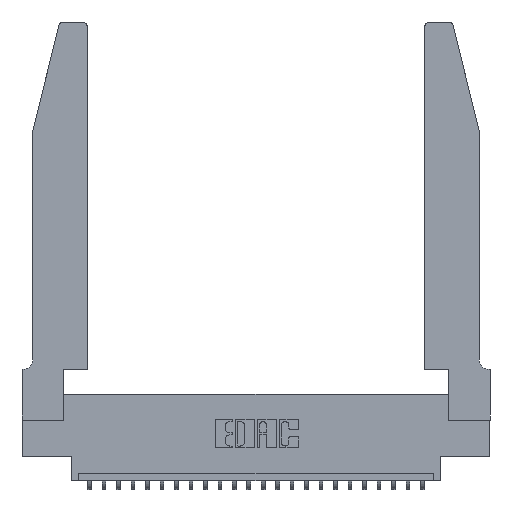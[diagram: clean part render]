
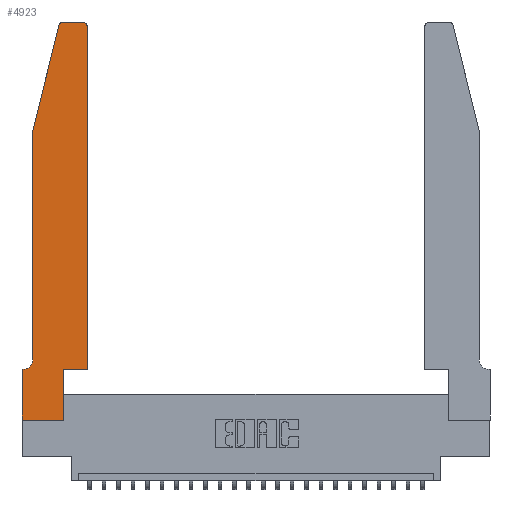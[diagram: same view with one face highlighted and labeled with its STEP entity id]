
A CAD part, top view. The second image highlights one B-rep face of the part: STEP entity #4923.
In plain terms, the highlighted planar face has unit normal (0, 0, 1).
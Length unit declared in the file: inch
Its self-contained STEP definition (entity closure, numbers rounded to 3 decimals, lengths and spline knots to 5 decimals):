
#191 = VERTEX_POINT ( 'NONE', #4531 ) ;
#282 = ORIENTED_EDGE ( 'NONE', *, *, #14211, .T. ) ;
#309 = CARTESIAN_POINT ( 'NONE',  ( 0.284, 2.72, 0.37 ) ) ;
#685 = VERTEX_POINT ( 'NONE', #8182 ) ;
#1137 = CARTESIAN_POINT ( 'NONE',  ( 0.4505, 0.35, 0.37 ) ) ;
#1182 = VERTEX_POINT ( 'NONE', #21952 ) ;
#1491 = CARTESIAN_POINT ( 'NONE',  ( 0.25487, 2.72718, 0.37 ) ) ;
#1698 = CARTESIAN_POINT ( 'NONE',  ( 0.4505, 0.35, 0.37 ) ) ;
#2178 = ORIENTED_EDGE ( 'NONE', *, *, #23063, .T. ) ;
#2293 = DIRECTION ( 'NONE',  ( 1., 0., 0. ) ) ;
#2399 = DIRECTION ( 'NONE',  ( -0.239, -0.971, 0. ) ) ;
#2492 = EDGE_CURVE ( 'NONE', #14007, #6624, #25092, .T. ) ;
#2654 = AXIS2_PLACEMENT_3D ( 'NONE', #11198, #19302, #3486 ) ;
#2881 = DIRECTION ( 'NONE',  ( -1., 0., 0. ) ) ;
#3036 = ORIENTED_EDGE ( 'NONE', *, *, #6409, .T. ) ;
#3486 = DIRECTION ( 'NONE',  ( 1., 0., 0. ) ) ;
#3730 = CIRCLE ( 'NONE', #21318, 0.03 ) ;
#4448 = DIRECTION ( 'NONE',  ( 0., 0., 1. ) ) ;
#4531 = CARTESIAN_POINT ( 'NONE',  ( 0.0755, 0.42, 0.37 ) ) ;
#4923 = ADVANCED_FACE ( 'NONE', ( #9296 ), #25029, .T. ) ;
#5009 = CARTESIAN_POINT ( 'NONE',  ( 0.0055, 0.42, 0.37 ) ) ;
#5676 = EDGE_CURVE ( 'NONE', #8826, #8177, #3730, .T. ) ;
#5836 = VERTEX_POINT ( 'NONE', #19314 ) ;
#6195 = DIRECTION ( 'NONE',  ( 0., 0., 1. ) ) ;
#6409 = EDGE_CURVE ( 'NONE', #7319, #21536, #24870, .T. ) ;
#6624 = VERTEX_POINT ( 'NONE', #1491 ) ;
#7091 = CARTESIAN_POINT ( 'NONE',  ( 0., 0.35, 0.37 ) ) ;
#7319 = VERTEX_POINT ( 'NONE', #7091 ) ;
#7355 = EDGE_LOOP ( 'NONE', ( #13079, #23089, #7685, #14093, #282, #2178, #3036, #17144, #7755, #24000, #13424, #10291 ) ) ;
#7619 = VECTOR ( 'NONE', #20845, 39.37008 ) ;
#7685 = ORIENTED_EDGE ( 'NONE', *, *, #12689, .T. ) ;
#7755 = ORIENTED_EDGE ( 'NONE', *, *, #13783, .T. ) ;
#7834 = DIRECTION ( 'NONE',  ( 0., 1., 0. ) ) ;
#8177 = VERTEX_POINT ( 'NONE', #15649 ) ;
#8182 = CARTESIAN_POINT ( 'NONE',  ( 0.4505, 0.35, 0.37 ) ) ;
#8200 = LINE ( 'NONE', #14822, #7619 ) ;
#8657 = EDGE_CURVE ( 'NONE', #1182, #685, #18036, .T. ) ;
#8658 = EDGE_CURVE ( 'NONE', #11736, #191, #8200, .T. ) ;
#8808 = LINE ( 'NONE', #13208, #17438 ) ;
#8826 = VERTEX_POINT ( 'NONE', #10407 ) ;
#9296 = FACE_OUTER_BOUND ( 'NONE', #7355, .T. ) ;
#10266 = CARTESIAN_POINT ( 'NONE',  ( 0.0055, 0.35, 0.37 ) ) ;
#10291 = ORIENTED_EDGE ( 'NONE', *, *, #5676, .T. ) ;
#10407 = CARTESIAN_POINT ( 'NONE',  ( 0.4505, 2.72, 0.37 ) ) ;
#10424 = VECTOR ( 'NONE', #2399, 39.37008 ) ;
#10442 = EDGE_CURVE ( 'NONE', #21536, #5836, #17632, .T. ) ;
#10556 = DIRECTION ( 'NONE',  ( 0., 0., -1. ) ) ;
#10636 = DIRECTION ( 'NONE',  ( -1., 0., 0. ) ) ;
#10854 = VECTOR ( 'NONE', #20711, 39.37008 ) ;
#11198 = CARTESIAN_POINT ( 'NONE',  ( 0., 0.35, 0.37 ) ) ;
#11328 = DIRECTION ( 'NONE',  ( -1., 0., 0. ) ) ;
#11674 = LINE ( 'NONE', #14182, #10424 ) ;
#11736 = VERTEX_POINT ( 'NONE', #25125 ) ;
#12235 = EDGE_CURVE ( 'NONE', #685, #8826, #17545, .T. ) ;
#12417 = DIRECTION ( 'NONE',  ( 1., 0., 0. ) ) ;
#12638 = DIRECTION ( 'NONE',  ( 1., 0., 0. ) ) ;
#12663 = CARTESIAN_POINT ( 'NONE',  ( 0.2605, 2.75, 0.37 ) ) ;
#12689 = EDGE_CURVE ( 'NONE', #6624, #11736, #11674, .T. ) ;
#12790 = VECTOR ( 'NONE', #12638, 39.37008 ) ;
#13079 = ORIENTED_EDGE ( 'NONE', *, *, #19976, .T. ) ;
#13208 = CARTESIAN_POINT ( 'NONE',  ( 0.0755, 0.35, 0.37 ) ) ;
#13424 = ORIENTED_EDGE ( 'NONE', *, *, #12235, .T. ) ;
#13458 = CARTESIAN_POINT ( 'NONE',  ( 0., 0., 0.37 ) ) ;
#13783 = EDGE_CURVE ( 'NONE', #5836, #1182, #22099, .T. ) ;
#14007 = VERTEX_POINT ( 'NONE', #21181 ) ;
#14093 = ORIENTED_EDGE ( 'NONE', *, *, #8658, .T. ) ;
#14182 = CARTESIAN_POINT ( 'NONE',  ( 0.0755, 2., 0.37 ) ) ;
#14195 = DIRECTION ( 'NONE',  ( 0., -1., 0. ) ) ;
#14211 = EDGE_CURVE ( 'NONE', #191, #19832, #19312, .T. ) ;
#14822 = CARTESIAN_POINT ( 'NONE',  ( 0.0755, 2., 0.37 ) ) ;
#15649 = CARTESIAN_POINT ( 'NONE',  ( 0.4205, 2.75, 0.37 ) ) ;
#16244 = DIRECTION ( 'NONE',  ( 0., 1., 0. ) ) ;
#16439 = AXIS2_PLACEMENT_3D ( 'NONE', #309, #4448, #2293 ) ;
#16747 = CARTESIAN_POINT ( 'NONE',  ( 0., 0., 0.37 ) ) ;
#17144 = ORIENTED_EDGE ( 'NONE', *, *, #10442, .T. ) ;
#17438 = VECTOR ( 'NONE', #11328, 39.37008 ) ;
#17545 = LINE ( 'NONE', #1698, #22488 ) ;
#17632 = LINE ( 'NONE', #16747, #10854 ) ;
#17854 = CARTESIAN_POINT ( 'NONE',  ( 0.2865, 0.35, 0.37 ) ) ;
#18036 = LINE ( 'NONE', #1137, #12790 ) ;
#18705 = VECTOR ( 'NONE', #16244, 39.37008 ) ;
#18734 = VECTOR ( 'NONE', #2881, 39.37008 ) ;
#19302 = DIRECTION ( 'NONE',  ( 0., 0., 1. ) ) ;
#19312 = CIRCLE ( 'NONE', #20579, 0.07 ) ;
#19314 = CARTESIAN_POINT ( 'NONE',  ( 0.2865, 0., 0.37 ) ) ;
#19658 = VECTOR ( 'NONE', #14195, 39.37008 ) ;
#19832 = VERTEX_POINT ( 'NONE', #10266 ) ;
#19976 = EDGE_CURVE ( 'NONE', #8177, #14007, #23934, .T. ) ;
#20579 = AXIS2_PLACEMENT_3D ( 'NONE', #5009, #10556, #10636 ) ;
#20711 = DIRECTION ( 'NONE',  ( 1., 0., 0. ) ) ;
#20845 = DIRECTION ( 'NONE',  ( 0., -1., 0. ) ) ;
#21181 = CARTESIAN_POINT ( 'NONE',  ( 0.284, 2.75, 0.37 ) ) ;
#21318 = AXIS2_PLACEMENT_3D ( 'NONE', #22100, #6195, #12417 ) ;
#21536 = VERTEX_POINT ( 'NONE', #13458 ) ;
#21952 = CARTESIAN_POINT ( 'NONE',  ( 0.2865, 0.35, 0.37 ) ) ;
#22099 = LINE ( 'NONE', #17854, #18705 ) ;
#22100 = CARTESIAN_POINT ( 'NONE',  ( 0.4205, 2.72, 0.37 ) ) ;
#22140 = CARTESIAN_POINT ( 'NONE',  ( 0., 0., 0.37 ) ) ;
#22488 = VECTOR ( 'NONE', #7834, 39.37008 ) ;
#23063 = EDGE_CURVE ( 'NONE', #19832, #7319, #8808, .T. ) ;
#23089 = ORIENTED_EDGE ( 'NONE', *, *, #2492, .T. ) ;
#23934 = LINE ( 'NONE', #12663, #18734 ) ;
#24000 = ORIENTED_EDGE ( 'NONE', *, *, #8657, .T. ) ;
#24870 = LINE ( 'NONE', #22140, #19658 ) ;
#25029 = PLANE ( 'NONE',  #2654 ) ;
#25092 = CIRCLE ( 'NONE', #16439, 0.03 ) ;
#25125 = CARTESIAN_POINT ( 'NONE',  ( 0.0755, 2., 0.37 ) ) ;
